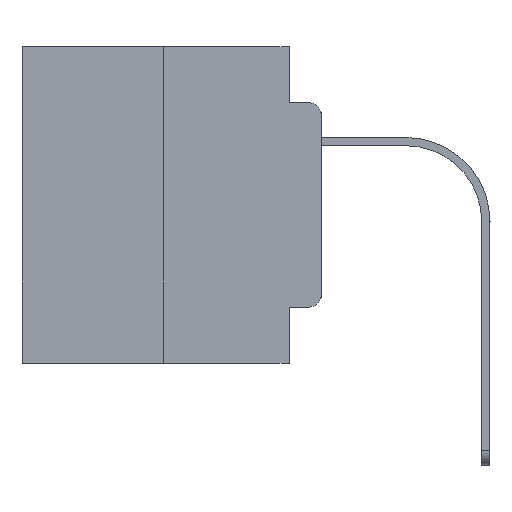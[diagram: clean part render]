
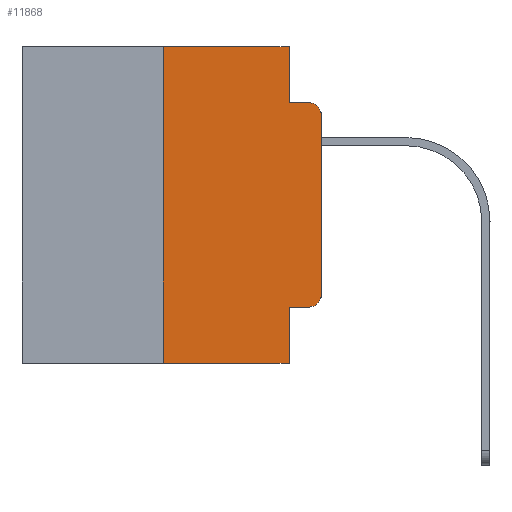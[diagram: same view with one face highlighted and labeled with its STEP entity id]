
A CAD part, left-side view. The second image highlights one B-rep face of the part: STEP entity #11868.
In plain terms, the highlighted planar face has unit normal (-1, 0, 0).
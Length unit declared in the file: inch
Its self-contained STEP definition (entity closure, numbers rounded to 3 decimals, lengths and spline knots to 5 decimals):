
#80 = EDGE_CURVE ( 'NONE', #4595, #25680, #17213, .T. ) ;
#721 = CARTESIAN_POINT ( 'NONE',  ( 0., 0., 0. ) ) ;
#752 = CIRCLE ( 'NONE', #16621, 0.02 ) ;
#1172 = EDGE_LOOP ( 'NONE', ( #9614, #12833, #7210, #19175, #24573, #3196, #24378, #1847, #18253, #2218 ) ) ;
#1655 = CARTESIAN_POINT ( 'NONE',  ( 0., 0.02, -0.0885 ) ) ;
#1796 = CARTESIAN_POINT ( 'NONE',  ( 0., 0.051, 0. ) ) ;
#1847 = ORIENTED_EDGE ( 'NONE', *, *, #8005, .F. ) ;
#2036 = EDGE_CURVE ( 'NONE', #23312, #17552, #24641, .T. ) ;
#2218 = ORIENTED_EDGE ( 'NONE', *, *, #23669, .T. ) ;
#2295 = VECTOR ( 'NONE', #9255, 39.37008 ) ;
#2313 = DIRECTION ( 'NONE',  ( 0., 0., 1. ) ) ;
#2622 = CIRCLE ( 'NONE', #13079, 0.02 ) ;
#2645 = VECTOR ( 'NONE', #14028, 39.37008 ) ;
#3196 = ORIENTED_EDGE ( 'NONE', *, *, #25468, .F. ) ;
#3256 = VECTOR ( 'NONE', #2313, 39.37008 ) ;
#4045 = DIRECTION ( 'NONE',  ( 1., 0., 0. ) ) ;
#4563 = DIRECTION ( 'NONE',  ( 0., 0., -1. ) ) ;
#4595 = VERTEX_POINT ( 'NONE', #12283 ) ;
#4603 = DIRECTION ( 'NONE',  ( -1., 0., 0. ) ) ;
#4656 = DIRECTION ( 'NONE',  ( 0., 0., -1. ) ) ;
#5211 = CARTESIAN_POINT ( 'NONE',  ( 0., 0.051, -0.0885 ) ) ;
#5299 = EDGE_CURVE ( 'NONE', #6990, #24316, #5935, .T. ) ;
#5304 = DIRECTION ( 'NONE',  ( 0., 0., -1. ) ) ;
#5570 = DIRECTION ( 'NONE',  ( 0., -1., 0. ) ) ;
#5935 = LINE ( 'NONE', #17553, #2645 ) ;
#6672 = VERTEX_POINT ( 'NONE', #17824 ) ;
#6747 = CARTESIAN_POINT ( 'NONE',  ( 0., 0.02, -0.1085 ) ) ;
#6934 = VECTOR ( 'NONE', #5570, 39.37008 ) ;
#6990 = VERTEX_POINT ( 'NONE', #24856 ) ;
#7130 = LINE ( 'NONE', #15226, #12732 ) ;
#7210 = ORIENTED_EDGE ( 'NONE', *, *, #80, .F. ) ;
#8005 = EDGE_CURVE ( 'NONE', #15476, #6672, #7130, .T. ) ;
#8909 = CARTESIAN_POINT ( 'NONE',  ( 0., 0.02, -0.3915 ) ) ;
#9128 = CARTESIAN_POINT ( 'NONE',  ( 0., 0., -0.1085 ) ) ;
#9255 = DIRECTION ( 'NONE',  ( 0., -1., 0. ) ) ;
#9351 = VERTEX_POINT ( 'NONE', #19580 ) ;
#9614 = ORIENTED_EDGE ( 'NONE', *, *, #2036, .T. ) ;
#9680 = LINE ( 'NONE', #15550, #16576 ) ;
#11291 = CARTESIAN_POINT ( 'NONE',  ( 0., 0., -0.3915 ) ) ;
#11560 = CARTESIAN_POINT ( 'NONE',  ( 0., 0.473, -0.5 ) ) ;
#11868 = ADVANCED_FACE ( 'NONE', ( #16571 ), #12149, .F. ) ;
#12149 = PLANE ( 'NONE',  #12258 ) ;
#12258 = AXIS2_PLACEMENT_3D ( 'NONE', #21934, #4045, #4563 ) ;
#12283 = CARTESIAN_POINT ( 'NONE',  ( 0., 0.051, -0.0885 ) ) ;
#12388 = EDGE_CURVE ( 'NONE', #17552, #25680, #2622, .T. ) ;
#12574 = DIRECTION ( 'NONE',  ( 0., 0., -1. ) ) ;
#12732 = VECTOR ( 'NONE', #5304, 39.37008 ) ;
#12764 = LINE ( 'NONE', #14348, #14145 ) ;
#12833 = ORIENTED_EDGE ( 'NONE', *, *, #12388, .T. ) ;
#13079 = AXIS2_PLACEMENT_3D ( 'NONE', #6747, #14833, #4656 ) ;
#13344 = VECTOR ( 'NONE', #15789, 39.37008 ) ;
#14028 = DIRECTION ( 'NONE',  ( 0., -1., 0. ) ) ;
#14145 = VECTOR ( 'NONE', #20475, 39.37008 ) ;
#14348 = CARTESIAN_POINT ( 'NONE',  ( 0., 0.25, 0. ) ) ;
#14833 = DIRECTION ( 'NONE',  ( -1., 0., 0. ) ) ;
#15226 = CARTESIAN_POINT ( 'NONE',  ( 0., 0.051, 0. ) ) ;
#15476 = VERTEX_POINT ( 'NONE', #21580 ) ;
#15550 = CARTESIAN_POINT ( 'NONE',  ( 0., 0.051, 0. ) ) ;
#15608 = LINE ( 'NONE', #11560, #6934 ) ;
#15789 = DIRECTION ( 'NONE',  ( 0., -1., 0. ) ) ;
#15860 = EDGE_CURVE ( 'NONE', #24316, #4595, #9680, .T. ) ;
#16069 = VERTEX_POINT ( 'NONE', #20607 ) ;
#16571 = FACE_OUTER_BOUND ( 'NONE', #1172, .T. ) ;
#16576 = VECTOR ( 'NONE', #25596, 39.37008 ) ;
#16621 = AXIS2_PLACEMENT_3D ( 'NONE', #8909, #4603, #12574 ) ;
#17213 = LINE ( 'NONE', #5211, #2295 ) ;
#17552 = VERTEX_POINT ( 'NONE', #9128 ) ;
#17553 = CARTESIAN_POINT ( 'NONE',  ( 0., 0.473, 0. ) ) ;
#17824 = CARTESIAN_POINT ( 'NONE',  ( 0., 0.051, -0.5 ) ) ;
#18253 = ORIENTED_EDGE ( 'NONE', *, *, #19431, .T. ) ;
#19175 = ORIENTED_EDGE ( 'NONE', *, *, #15860, .F. ) ;
#19431 = EDGE_CURVE ( 'NONE', #15476, #16069, #23393, .T. ) ;
#19580 = CARTESIAN_POINT ( 'NONE',  ( 0., 0.25, -0.5 ) ) ;
#20475 = DIRECTION ( 'NONE',  ( 0., 0., 1. ) ) ;
#20607 = CARTESIAN_POINT ( 'NONE',  ( 0., 0.02, -0.4115 ) ) ;
#21446 = EDGE_CURVE ( 'NONE', #9351, #6672, #15608, .T. ) ;
#21580 = CARTESIAN_POINT ( 'NONE',  ( 0., 0.051, -0.4115 ) ) ;
#21934 = CARTESIAN_POINT ( 'NONE',  ( 0., 0.473, 0. ) ) ;
#23312 = VERTEX_POINT ( 'NONE', #11291 ) ;
#23393 = LINE ( 'NONE', #25332, #13344 ) ;
#23669 = EDGE_CURVE ( 'NONE', #16069, #23312, #752, .T. ) ;
#24316 = VERTEX_POINT ( 'NONE', #1796 ) ;
#24378 = ORIENTED_EDGE ( 'NONE', *, *, #21446, .T. ) ;
#24573 = ORIENTED_EDGE ( 'NONE', *, *, #5299, .F. ) ;
#24641 = LINE ( 'NONE', #721, #3256 ) ;
#24856 = CARTESIAN_POINT ( 'NONE',  ( 0., 0.25, 0. ) ) ;
#25332 = CARTESIAN_POINT ( 'NONE',  ( 0., 0.051, -0.4115 ) ) ;
#25468 = EDGE_CURVE ( 'NONE', #9351, #6990, #12764, .T. ) ;
#25596 = DIRECTION ( 'NONE',  ( 0., 0., -1. ) ) ;
#25680 = VERTEX_POINT ( 'NONE', #1655 ) ;
